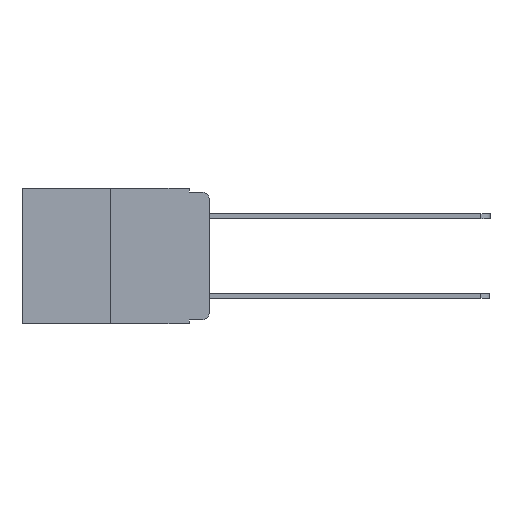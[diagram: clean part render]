
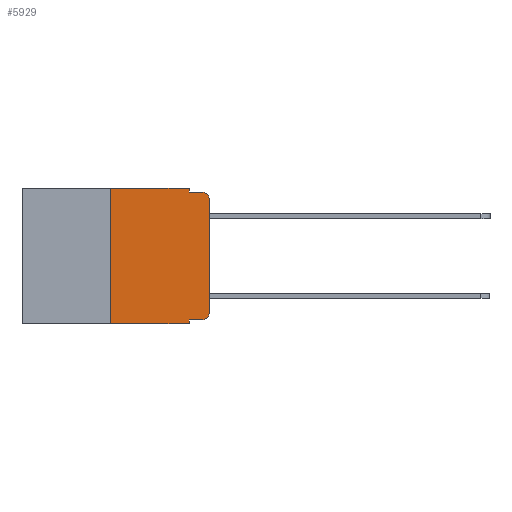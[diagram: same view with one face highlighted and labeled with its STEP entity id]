
A CAD part, left-side view. The second image highlights one B-rep face of the part: STEP entity #5929.
In plain terms, the highlighted planar face has unit normal (-1, 0, 0).
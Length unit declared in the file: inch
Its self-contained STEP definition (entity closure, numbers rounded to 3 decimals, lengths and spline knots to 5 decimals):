
#301 = DIRECTION ( 'NONE',  ( 0., 0., -1. ) ) ;
#381 = DIRECTION ( 'NONE',  ( -1., 0., 0. ) ) ;
#537 = DIRECTION ( 'NONE',  ( 0., -1., 0. ) ) ;
#702 = VERTEX_POINT ( 'NONE', #7707 ) ;
#1458 = CARTESIAN_POINT ( 'NONE',  ( 0., 0.051, -0.01 ) ) ;
#1812 = DIRECTION ( 'NONE',  ( 0., -1., 0. ) ) ;
#2036 = CARTESIAN_POINT ( 'NONE',  ( 0., 0.051, 0. ) ) ;
#2382 = VERTEX_POINT ( 'NONE', #8458 ) ;
#2478 = EDGE_CURVE ( 'NONE', #2382, #14272, #8148, .T. ) ;
#2482 = VERTEX_POINT ( 'NONE', #1458 ) ;
#2681 = ORIENTED_EDGE ( 'NONE', *, *, #15379, .F. ) ;
#3548 = ORIENTED_EDGE ( 'NONE', *, *, #2478, .T. ) ;
#3625 = DIRECTION ( 'NONE',  ( 1., 0., 0. ) ) ;
#3728 = VECTOR ( 'NONE', #7844, 39.37008 ) ;
#3760 = LINE ( 'NONE', #7697, #7655 ) ;
#4223 = DIRECTION ( 'NONE',  ( 0., 0., -1. ) ) ;
#5636 = CARTESIAN_POINT ( 'NONE',  ( 0., 0.051, 0. ) ) ;
#5929 = ADVANCED_FACE ( 'NONE', ( #16162 ), #11831, .F. ) ;
#6193 = DIRECTION ( 'NONE',  ( 0., 0., 1. ) ) ;
#6325 = CARTESIAN_POINT ( 'NONE',  ( 0., 0.25, 0. ) ) ;
#6495 = ORIENTED_EDGE ( 'NONE', *, *, #13260, .T. ) ;
#6708 = CARTESIAN_POINT ( 'NONE',  ( 0., 0.051, -0.333 ) ) ;
#6781 = AXIS2_PLACEMENT_3D ( 'NONE', #10553, #381, #12139 ) ;
#7494 = VERTEX_POINT ( 'NONE', #6708 ) ;
#7655 = VECTOR ( 'NONE', #9340, 39.37008 ) ;
#7693 = CARTESIAN_POINT ( 'NONE',  ( 0., 0.473, -0.343 ) ) ;
#7697 = CARTESIAN_POINT ( 'NONE',  ( 0., 0.051, -0.333 ) ) ;
#7707 = CARTESIAN_POINT ( 'NONE',  ( 0., 0., -0.313 ) ) ;
#7713 = CIRCLE ( 'NONE', #6781, 0.02 ) ;
#7844 = DIRECTION ( 'NONE',  ( 0., -1., 0. ) ) ;
#7951 = ORIENTED_EDGE ( 'NONE', *, *, #13149, .F. ) ;
#8148 = LINE ( 'NONE', #7693, #3728 ) ;
#8458 = CARTESIAN_POINT ( 'NONE',  ( 0., 0.25, -0.343 ) ) ;
#8870 = ORIENTED_EDGE ( 'NONE', *, *, #19373, .T. ) ;
#8922 = VERTEX_POINT ( 'NONE', #15302 ) ;
#9230 = DIRECTION ( 'NONE',  ( -1., 0., 0. ) ) ;
#9260 = ORIENTED_EDGE ( 'NONE', *, *, #14347, .T. ) ;
#9340 = DIRECTION ( 'NONE',  ( 0., -1., 0. ) ) ;
#9594 = ORIENTED_EDGE ( 'NONE', *, *, #20332, .T. ) ;
#10300 = LINE ( 'NONE', #13369, #18042 ) ;
#10553 = CARTESIAN_POINT ( 'NONE',  ( 0., 0.02, -0.313 ) ) ;
#10656 = CARTESIAN_POINT ( 'NONE',  ( 0., 0.051, -0.343 ) ) ;
#10692 = LINE ( 'NONE', #14201, #14407 ) ;
#10817 = VERTEX_POINT ( 'NONE', #2036 ) ;
#11312 = CARTESIAN_POINT ( 'NONE',  ( 0., 0.02, -0.01 ) ) ;
#11831 = PLANE ( 'NONE',  #13954 ) ;
#12111 = LINE ( 'NONE', #16878, #16289 ) ;
#12139 = DIRECTION ( 'NONE',  ( 0., 0., -1. ) ) ;
#12366 = CARTESIAN_POINT ( 'NONE',  ( 0., 0.051, 0. ) ) ;
#12418 = VECTOR ( 'NONE', #301, 39.37008 ) ;
#12819 = CIRCLE ( 'NONE', #13529, 0.02 ) ;
#13149 = EDGE_CURVE ( 'NONE', #16502, #10817, #10300, .T. ) ;
#13260 = EDGE_CURVE ( 'NONE', #8922, #702, #7713, .T. ) ;
#13369 = CARTESIAN_POINT ( 'NONE',  ( 0., 0.473, 0. ) ) ;
#13391 = CARTESIAN_POINT ( 'NONE',  ( 0., 0.473, 0. ) ) ;
#13529 = AXIS2_PLACEMENT_3D ( 'NONE', #18551, #9230, #20023 ) ;
#13843 = ORIENTED_EDGE ( 'NONE', *, *, #18370, .F. ) ;
#13954 = AXIS2_PLACEMENT_3D ( 'NONE', #13391, #3625, #15001 ) ;
#14201 = CARTESIAN_POINT ( 'NONE',  ( 0., 0.25, 0. ) ) ;
#14272 = VERTEX_POINT ( 'NONE', #10656 ) ;
#14347 = EDGE_CURVE ( 'NONE', #7494, #8922, #3760, .T. ) ;
#14407 = VECTOR ( 'NONE', #6193, 39.37008 ) ;
#14547 = LINE ( 'NONE', #18213, #18061 ) ;
#15001 = DIRECTION ( 'NONE',  ( 0., 0., -1. ) ) ;
#15302 = CARTESIAN_POINT ( 'NONE',  ( 0., 0.02, -0.333 ) ) ;
#15379 = EDGE_CURVE ( 'NONE', #7494, #14272, #16576, .T. ) ;
#15585 = LINE ( 'NONE', #12366, #16082 ) ;
#15698 = ORIENTED_EDGE ( 'NONE', *, *, #16419, .F. ) ;
#16082 = VECTOR ( 'NONE', #4223, 39.37008 ) ;
#16162 = FACE_OUTER_BOUND ( 'NONE', #17290, .T. ) ;
#16289 = VECTOR ( 'NONE', #537, 39.37008 ) ;
#16419 = EDGE_CURVE ( 'NONE', #2382, #16502, #10692, .T. ) ;
#16502 = VERTEX_POINT ( 'NONE', #6325 ) ;
#16576 = LINE ( 'NONE', #5636, #12418 ) ;
#16860 = VERTEX_POINT ( 'NONE', #20688 ) ;
#16878 = CARTESIAN_POINT ( 'NONE',  ( 0., 0.051, -0.01 ) ) ;
#17290 = EDGE_LOOP ( 'NONE', ( #9594, #8870, #13843, #18466, #7951, #15698, #3548, #2681, #9260, #6495 ) ) ;
#17374 = EDGE_CURVE ( 'NONE', #10817, #2482, #15585, .T. ) ;
#18042 = VECTOR ( 'NONE', #1812, 39.37008 ) ;
#18061 = VECTOR ( 'NONE', #18273, 39.37008 ) ;
#18213 = CARTESIAN_POINT ( 'NONE',  ( 0., 0., 0. ) ) ;
#18273 = DIRECTION ( 'NONE',  ( 0., 0., 1. ) ) ;
#18370 = EDGE_CURVE ( 'NONE', #2482, #19704, #12111, .T. ) ;
#18466 = ORIENTED_EDGE ( 'NONE', *, *, #17374, .F. ) ;
#18551 = CARTESIAN_POINT ( 'NONE',  ( 0., 0.02, -0.03 ) ) ;
#19373 = EDGE_CURVE ( 'NONE', #16860, #19704, #12819, .T. ) ;
#19704 = VERTEX_POINT ( 'NONE', #11312 ) ;
#20023 = DIRECTION ( 'NONE',  ( 0., 0., -1. ) ) ;
#20332 = EDGE_CURVE ( 'NONE', #702, #16860, #14547, .T. ) ;
#20688 = CARTESIAN_POINT ( 'NONE',  ( 0., 0., -0.03 ) ) ;
